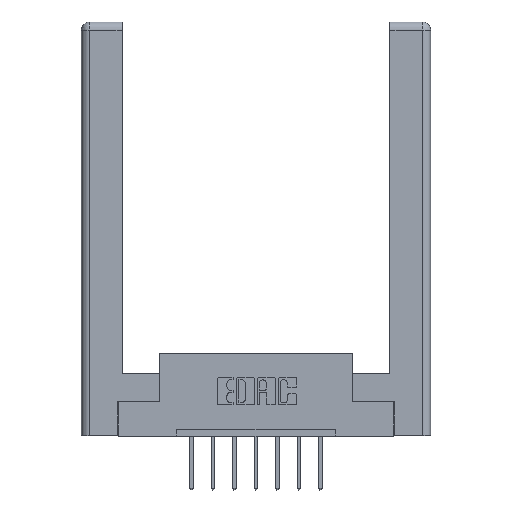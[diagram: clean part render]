
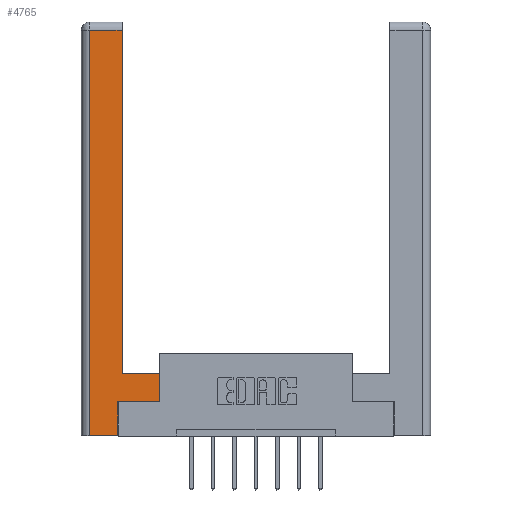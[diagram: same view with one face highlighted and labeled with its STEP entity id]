
A CAD part, top view. The second image highlights one B-rep face of the part: STEP entity #4765.
In plain terms, the highlighted planar face has unit normal (0, 0, 1).
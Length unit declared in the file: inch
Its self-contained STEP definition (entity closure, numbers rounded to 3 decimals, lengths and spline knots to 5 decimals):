
#895 = DIRECTION ( 'NONE',  ( 0., 1., 0. ) ) ;
#999 = CARTESIAN_POINT ( 'NONE',  ( 0.565, 0.45, 0. ) ) ;
#1369 = VERTEX_POINT ( 'NONE', #8307 ) ;
#1395 = DIRECTION ( 'NONE',  ( 0., -1., 0. ) ) ;
#1458 = EDGE_CURVE ( 'NONE', #5155, #6790, #11707, .T. ) ;
#1954 = CARTESIAN_POINT ( 'NONE',  ( 0.0615, 2.94, 0. ) ) ;
#2249 = PLANE ( 'NONE',  #7207 ) ;
#2613 = CARTESIAN_POINT ( 'NONE',  ( 0.295, 0.45, 0. ) ) ;
#2642 = LINE ( 'NONE', #2827, #8205 ) ;
#2722 = LINE ( 'NONE', #9176, #4517 ) ;
#2769 = DIRECTION ( 'NONE',  ( -1., 0., 0. ) ) ;
#2783 = ORIENTED_EDGE ( 'NONE', *, *, #8831, .T. ) ;
#2827 = CARTESIAN_POINT ( 'NONE',  ( 0.295, 0.45, 0. ) ) ;
#2913 = DIRECTION ( 'NONE',  ( 0., 1., 0. ) ) ;
#3168 = ORIENTED_EDGE ( 'NONE', *, *, #12199, .T. ) ;
#3186 = DIRECTION ( 'NONE',  ( 0., 0., -1. ) ) ;
#3421 = VECTOR ( 'NONE', #9158, 39.37008 ) ;
#3911 = LINE ( 'NONE', #9242, #7825 ) ;
#4033 = CARTESIAN_POINT ( 'NONE',  ( 0.0615, 2.94, 0. ) ) ;
#4168 = EDGE_CURVE ( 'NONE', #7870, #9048, #12332, .T. ) ;
#4445 = LINE ( 'NONE', #7116, #7928 ) ;
#4463 = VECTOR ( 'NONE', #2769, 39.37008 ) ;
#4517 = VECTOR ( 'NONE', #6315, 39.37008 ) ;
#4668 = CARTESIAN_POINT ( 'NONE',  ( 0.265, 0.245, 0. ) ) ;
#4765 = ADVANCED_FACE ( 'NONE', ( #6909 ), #2249, .F. ) ;
#5051 = EDGE_CURVE ( 'NONE', #6508, #5155, #9449, .T. ) ;
#5155 = VERTEX_POINT ( 'NONE', #8023 ) ;
#5200 = CARTESIAN_POINT ( 'NONE',  ( 0.565, 0.245, 0. ) ) ;
#5757 = CARTESIAN_POINT ( 'NONE',  ( 0.265, 0.245, 0. ) ) ;
#5813 = DIRECTION ( 'NONE',  ( -1., 0., 0. ) ) ;
#6045 = CARTESIAN_POINT ( 'NONE',  ( 0.265, 0., 0. ) ) ;
#6152 = EDGE_CURVE ( 'NONE', #6790, #1369, #4445, .T. ) ;
#6315 = DIRECTION ( 'NONE',  ( 1., 0., 0. ) ) ;
#6355 = ORIENTED_EDGE ( 'NONE', *, *, #11746, .T. ) ;
#6508 = VERTEX_POINT ( 'NONE', #2613 ) ;
#6790 = VERTEX_POINT ( 'NONE', #4033 ) ;
#6909 = FACE_OUTER_BOUND ( 'NONE', #9839, .T. ) ;
#7017 = DIRECTION ( 'NONE',  ( -1., 0., 0. ) ) ;
#7116 = CARTESIAN_POINT ( 'NONE',  ( 0.0615, 0., 0. ) ) ;
#7207 = AXIS2_PLACEMENT_3D ( 'NONE', #7858, #3186, #7017 ) ;
#7237 = CARTESIAN_POINT ( 'NONE',  ( 0.295, 3., 0. ) ) ;
#7290 = LINE ( 'NONE', #7496, #12403 ) ;
#7496 = CARTESIAN_POINT ( 'NONE',  ( 0.565, 0.45, 0. ) ) ;
#7825 = VECTOR ( 'NONE', #11277, 39.37008 ) ;
#7858 = CARTESIAN_POINT ( 'NONE',  ( 0., 0., 0. ) ) ;
#7870 = VERTEX_POINT ( 'NONE', #6045 ) ;
#7928 = VECTOR ( 'NONE', #1395, 39.37008 ) ;
#8011 = EDGE_CURVE ( 'NONE', #1369, #7870, #2722, .T. ) ;
#8023 = CARTESIAN_POINT ( 'NONE',  ( 0.295, 2.94, 0. ) ) ;
#8205 = VECTOR ( 'NONE', #5813, 39.37008 ) ;
#8307 = CARTESIAN_POINT ( 'NONE',  ( 0.0615, 0., 0. ) ) ;
#8783 = ORIENTED_EDGE ( 'NONE', *, *, #5051, .T. ) ;
#8831 = EDGE_CURVE ( 'NONE', #9048, #10076, #3911, .T. ) ;
#8911 = ORIENTED_EDGE ( 'NONE', *, *, #4168, .T. ) ;
#9048 = VERTEX_POINT ( 'NONE', #5757 ) ;
#9158 = DIRECTION ( 'NONE',  ( 0., 1., 0. ) ) ;
#9176 = CARTESIAN_POINT ( 'NONE',  ( 0.265, 0., 0. ) ) ;
#9242 = CARTESIAN_POINT ( 'NONE',  ( 0.565, 0.245, 0. ) ) ;
#9320 = VECTOR ( 'NONE', #2913, 39.37008 ) ;
#9449 = LINE ( 'NONE', #7237, #3421 ) ;
#9839 = EDGE_LOOP ( 'NONE', ( #8783, #10406, #10850, #10010, #8911, #2783, #3168, #6355 ) ) ;
#10010 = ORIENTED_EDGE ( 'NONE', *, *, #8011, .T. ) ;
#10076 = VERTEX_POINT ( 'NONE', #5200 ) ;
#10271 = VERTEX_POINT ( 'NONE', #999 ) ;
#10406 = ORIENTED_EDGE ( 'NONE', *, *, #1458, .T. ) ;
#10850 = ORIENTED_EDGE ( 'NONE', *, *, #6152, .T. ) ;
#11277 = DIRECTION ( 'NONE',  ( 1., 0., 0. ) ) ;
#11707 = LINE ( 'NONE', #1954, #4463 ) ;
#11746 = EDGE_CURVE ( 'NONE', #10271, #6508, #2642, .T. ) ;
#12199 = EDGE_CURVE ( 'NONE', #10076, #10271, #7290, .T. ) ;
#12332 = LINE ( 'NONE', #4668, #9320 ) ;
#12403 = VECTOR ( 'NONE', #895, 39.37008 ) ;
